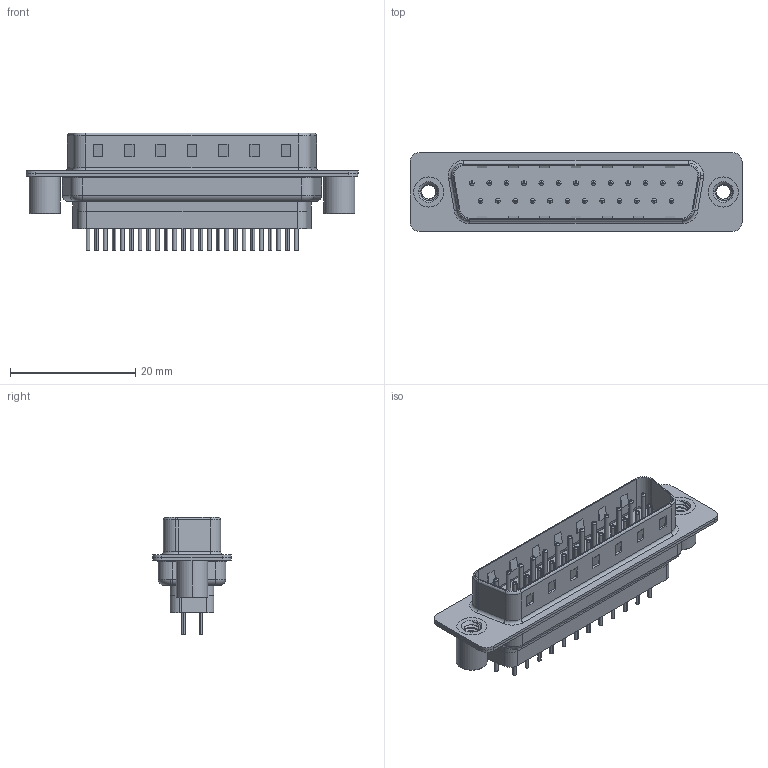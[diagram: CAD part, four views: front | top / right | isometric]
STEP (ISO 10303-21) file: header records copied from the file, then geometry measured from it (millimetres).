
FILE_DESCRIPTION (( 'STEP AP203' ), '1' );
FILE_NAME ('627-025-228-269.STEP', '2020-07-21T16:50:03', ( '' ), ( '' ), 'SwSTEP 2.0', 'SolidWorks 2020', '' );
FILE_SCHEMA (( 'CONFIG_CONTROL_DESIGN' ));
Length unit declared in the file: millimetre
Products named in the file (7): 627 Contact Row 2_28L; 627 Shell Front_25 Contacts; 627 4-40 Threaded Standoff BS; 627-025-228-269; 627 Contact Row 1_28L; 627 Housing_25 FF; 627 Shell Rear_25 Contacts
Assembly tree (30 placements, depth 2):
  627-025-228-269
    627 Housing_25 FF
    627 Shell Front_25 Contacts
    627 Shell Rear_25 Contacts
    627 Contact Row 1_28L  x13
    627 Contact Row 2_28L  x12
    627 4-40 Threaded Standoff BS  x2
Bounding box: 53 x 12.6 x 18.8 mm (x, y, z)
Volume: 3374.1 mm3; surface area: 9114.8 mm2
Topology: 31 solids, 31 shells, 2909 faces, 7623 edges, 4737 vertices
Faces by surface type: cylinder 1137, plane 777, torus 725, cone 264, bspline 6
Entity records: 27844 total; most frequent: CARTESIAN_POINT 6433, DIRECTION 4468, ORIENTED_EDGE 4010, EDGE_CURVE 2005, AXIS2_PLACEMENT_3D 1769, VERTEX_POINT 1283, EDGE_LOOP 996, CIRCLE 944
